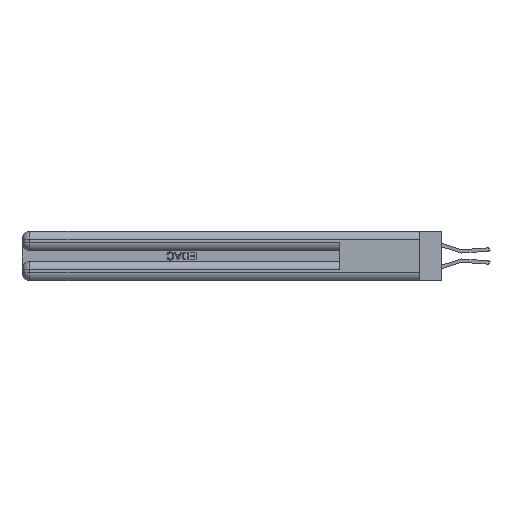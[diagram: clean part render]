
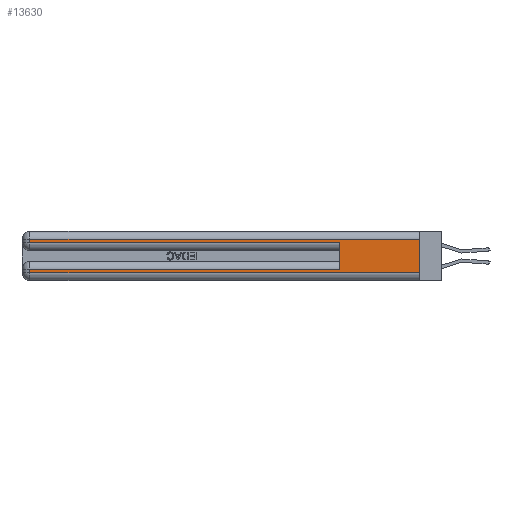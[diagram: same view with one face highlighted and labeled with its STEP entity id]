
A CAD part, left-side view. The second image highlights one B-rep face of the part: STEP entity #13630.
In plain terms, the highlighted planar face has unit normal (-1, 0, 0).
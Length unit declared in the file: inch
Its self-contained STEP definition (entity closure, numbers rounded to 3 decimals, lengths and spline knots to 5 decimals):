
#278 = CARTESIAN_POINT ( 'NONE',  ( 0., 2.94, 0.285 ) ) ;
#947 = VERTEX_POINT ( 'NONE', #14583 ) ;
#2283 = CARTESIAN_POINT ( 'NONE',  ( 0., 0., 0.37 ) ) ;
#2529 = CARTESIAN_POINT ( 'NONE',  ( 0., 0., 0.085 ) ) ;
#3028 = DIRECTION ( 'NONE',  ( 0., -1., 0. ) ) ;
#4936 = EDGE_CURVE ( 'NONE', #5881, #17292, #33964, .T. ) ;
#5128 = DIRECTION ( 'NONE',  ( 0., 0., -1. ) ) ;
#5720 = EDGE_CURVE ( 'NONE', #30953, #23725, #6215, .T. ) ;
#5833 = FACE_OUTER_BOUND ( 'NONE', #35757, .T. ) ;
#5881 = VERTEX_POINT ( 'NONE', #22146 ) ;
#6215 = LINE ( 'NONE', #21506, #38623 ) ;
#7036 = VECTOR ( 'NONE', #27679, 39.37008 ) ;
#7727 = LINE ( 'NONE', #17145, #15891 ) ;
#7913 = LINE ( 'NONE', #16536, #23214 ) ;
#8145 = ORIENTED_EDGE ( 'NONE', *, *, #38167, .F. ) ;
#8374 = EDGE_CURVE ( 'NONE', #17292, #30953, #29550, .T. ) ;
#8552 = CARTESIAN_POINT ( 'NONE',  ( 0., 0., 0.37 ) ) ;
#9718 = VECTOR ( 'NONE', #30204, 39.37008 ) ;
#10177 = VECTOR ( 'NONE', #34276, 39.37008 ) ;
#11667 = DIRECTION ( 'NONE',  ( 1., 0., 0. ) ) ;
#12038 = ORIENTED_EDGE ( 'NONE', *, *, #5720, .T. ) ;
#12128 = EDGE_CURVE ( 'NONE', #34434, #23725, #25120, .T. ) ;
#13072 = CARTESIAN_POINT ( 'NONE',  ( 0., 0., 0.285 ) ) ;
#13630 = ADVANCED_FACE ( 'NONE', ( #5833 ), #26837, .F. ) ;
#14493 = AXIS2_PLACEMENT_3D ( 'NONE', #8552, #11667, #32906 ) ;
#14583 = CARTESIAN_POINT ( 'NONE',  ( 0., 2.94, 0.31 ) ) ;
#15119 = VERTEX_POINT ( 'NONE', #278 ) ;
#15280 = VECTOR ( 'NONE', #5128, 39.37008 ) ;
#15571 = VERTEX_POINT ( 'NONE', #32914 ) ;
#15891 = VECTOR ( 'NONE', #26323, 39.37008 ) ;
#16536 = CARTESIAN_POINT ( 'NONE',  ( 0., 0., 0.31 ) ) ;
#16569 = CARTESIAN_POINT ( 'NONE',  ( 0., 2.94, 0.06 ) ) ;
#17145 = CARTESIAN_POINT ( 'NONE',  ( 0., 0.6, 0.145 ) ) ;
#17292 = VERTEX_POINT ( 'NONE', #27531 ) ;
#17725 = DIRECTION ( 'NONE',  ( 0., 0., -1. ) ) ;
#18667 = ORIENTED_EDGE ( 'NONE', *, *, #12128, .F. ) ;
#20583 = ORIENTED_EDGE ( 'NONE', *, *, #35239, .T. ) ;
#21506 = CARTESIAN_POINT ( 'NONE',  ( 0., 0., 0.06 ) ) ;
#22052 = CARTESIAN_POINT ( 'NONE',  ( 0., 0., 0.06 ) ) ;
#22146 = CARTESIAN_POINT ( 'NONE',  ( 0., 0.6, 0.085 ) ) ;
#23214 = VECTOR ( 'NONE', #25579, 39.37008 ) ;
#23355 = LINE ( 'NONE', #36630, #7036 ) ;
#23512 = CARTESIAN_POINT ( 'NONE',  ( 0., 2.94, 0.37 ) ) ;
#23725 = VERTEX_POINT ( 'NONE', #22052 ) ;
#24171 = VECTOR ( 'NONE', #17725, 39.37008 ) ;
#24578 = CARTESIAN_POINT ( 'NONE',  ( 0., 0., 0.31 ) ) ;
#25109 = EDGE_CURVE ( 'NONE', #15119, #15571, #33488, .T. ) ;
#25120 = LINE ( 'NONE', #2283, #24171 ) ;
#25353 = ORIENTED_EDGE ( 'NONE', *, *, #4936, .T. ) ;
#25579 = DIRECTION ( 'NONE',  ( 0., 1., 0. ) ) ;
#26323 = DIRECTION ( 'NONE',  ( 0., 0., 1. ) ) ;
#26837 = PLANE ( 'NONE',  #14493 ) ;
#27531 = CARTESIAN_POINT ( 'NONE',  ( 0., 2.94, 0.085 ) ) ;
#27679 = DIRECTION ( 'NONE',  ( 0., 0., -1. ) ) ;
#28270 = EDGE_CURVE ( 'NONE', #947, #15119, #23355, .T. ) ;
#29550 = LINE ( 'NONE', #23512, #15280 ) ;
#30204 = DIRECTION ( 'NONE',  ( 0., 1., 0. ) ) ;
#30953 = VERTEX_POINT ( 'NONE', #16569 ) ;
#31499 = ORIENTED_EDGE ( 'NONE', *, *, #25109, .T. ) ;
#32906 = DIRECTION ( 'NONE',  ( 0., 0., -1. ) ) ;
#32914 = CARTESIAN_POINT ( 'NONE',  ( 0., 0.6, 0.285 ) ) ;
#33405 = ORIENTED_EDGE ( 'NONE', *, *, #8374, .T. ) ;
#33488 = LINE ( 'NONE', #13072, #10177 ) ;
#33964 = LINE ( 'NONE', #2529, #9718 ) ;
#34276 = DIRECTION ( 'NONE',  ( 0., -1., 0. ) ) ;
#34434 = VERTEX_POINT ( 'NONE', #24578 ) ;
#35239 = EDGE_CURVE ( 'NONE', #34434, #947, #7913, .T. ) ;
#35757 = EDGE_LOOP ( 'NONE', ( #18667, #20583, #36688, #31499, #8145, #25353, #33405, #12038 ) ) ;
#36630 = CARTESIAN_POINT ( 'NONE',  ( 0., 2.94, 0.37 ) ) ;
#36688 = ORIENTED_EDGE ( 'NONE', *, *, #28270, .T. ) ;
#38167 = EDGE_CURVE ( 'NONE', #5881, #15571, #7727, .T. ) ;
#38623 = VECTOR ( 'NONE', #3028, 39.37008 ) ;
